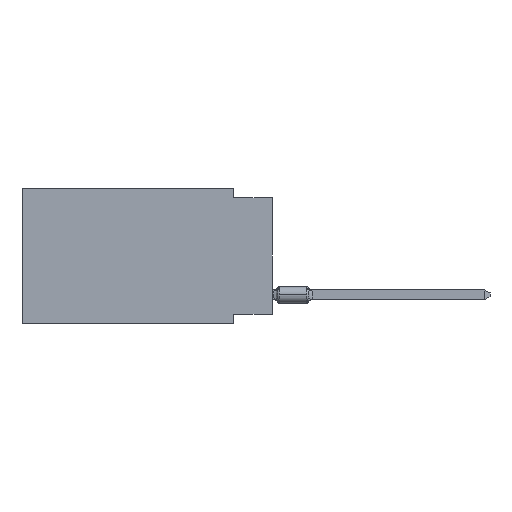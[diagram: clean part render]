
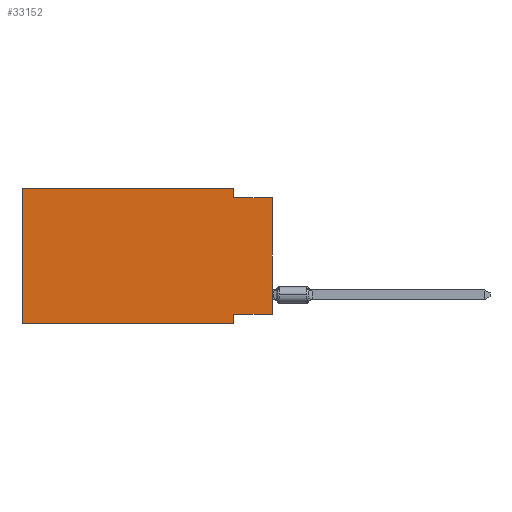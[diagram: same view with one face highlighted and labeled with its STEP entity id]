
A CAD part, left-side view. The second image highlights one B-rep face of the part: STEP entity #33152.
In plain terms, the highlighted planar face has unit normal (-1, 0, 0).
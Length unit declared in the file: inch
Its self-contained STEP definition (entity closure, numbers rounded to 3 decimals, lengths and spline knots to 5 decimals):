
#201 = VERTEX_POINT ( 'NONE', #7685 ) ;
#712 = DIRECTION ( 'NONE',  ( 0., 0., -1. ) ) ;
#1995 = EDGE_CURVE ( 'NONE', #35652, #3189, #28997, .T. ) ;
#3189 = VERTEX_POINT ( 'NONE', #18031 ) ;
#3598 = FACE_OUTER_BOUND ( 'NONE', #28103, .T. ) ;
#4036 = DIRECTION ( 'NONE',  ( 0., 0., 1. ) ) ;
#6477 = EDGE_CURVE ( 'NONE', #38400, #25236, #16079, .T. ) ;
#6953 = DIRECTION ( 'NONE',  ( 0., 0., -1. ) ) ;
#7001 = CARTESIAN_POINT ( 'NONE',  ( 0., 0.1, -0.35 ) ) ;
#7685 = CARTESIAN_POINT ( 'NONE',  ( 0., 0., -0.025 ) ) ;
#8090 = LINE ( 'NONE', #29422, #22528 ) ;
#8241 = VECTOR ( 'NONE', #712, 39.37008 ) ;
#9896 = PLANE ( 'NONE',  #38594 ) ;
#12372 = CARTESIAN_POINT ( 'NONE',  ( 0., 0.1, -0.025 ) ) ;
#12717 = DIRECTION ( 'NONE',  ( 0., -1., 0. ) ) ;
#12988 = CARTESIAN_POINT ( 'NONE',  ( 0., 0.645, 0. ) ) ;
#15323 = EDGE_CURVE ( 'NONE', #38400, #37860, #37499, .T. ) ;
#15600 = ORIENTED_EDGE ( 'NONE', *, *, #6477, .T. ) ;
#15700 = EDGE_CURVE ( 'NONE', #3189, #25236, #27212, .T. ) ;
#16079 = LINE ( 'NONE', #29769, #20965 ) ;
#16549 = ORIENTED_EDGE ( 'NONE', *, *, #17083, .F. ) ;
#17083 = EDGE_CURVE ( 'NONE', #25740, #201, #8090, .T. ) ;
#18031 = CARTESIAN_POINT ( 'NONE',  ( 0., 0.1, -0.325 ) ) ;
#18383 = VECTOR ( 'NONE', #39969, 39.37008 ) ;
#18603 = CARTESIAN_POINT ( 'NONE',  ( 0., 0.1, 0. ) ) ;
#18643 = DIRECTION ( 'NONE',  ( 0., -1., 0. ) ) ;
#19701 = EDGE_CURVE ( 'NONE', #35652, #201, #42892, .T. ) ;
#20965 = VECTOR ( 'NONE', #12717, 39.37008 ) ;
#22006 = EDGE_CURVE ( 'NONE', #24143, #25740, #39508, .T. ) ;
#22528 = VECTOR ( 'NONE', #18643, 39.37008 ) ;
#22615 = LINE ( 'NONE', #12988, #33573 ) ;
#24143 = VERTEX_POINT ( 'NONE', #18603 ) ;
#24515 = CARTESIAN_POINT ( 'NONE',  ( 0., 0.645, -0.35 ) ) ;
#25206 = CARTESIAN_POINT ( 'NONE',  ( 0., 0.1, -0.35 ) ) ;
#25236 = VERTEX_POINT ( 'NONE', #25206 ) ;
#25554 = DIRECTION ( 'NONE',  ( 0., 0., -1. ) ) ;
#25740 = VERTEX_POINT ( 'NONE', #12372 ) ;
#26337 = VECTOR ( 'NONE', #25554, 39.37008 ) ;
#26665 = DIRECTION ( 'NONE',  ( 0., -1., 0. ) ) ;
#27212 = LINE ( 'NONE', #7001, #8241 ) ;
#28103 = EDGE_LOOP ( 'NONE', ( #37641, #16549, #42723, #44230, #43222, #15600, #42569, #43515 ) ) ;
#28997 = LINE ( 'NONE', #36186, #42682 ) ;
#29422 = CARTESIAN_POINT ( 'NONE',  ( 0., 0., -0.025 ) ) ;
#29769 = CARTESIAN_POINT ( 'NONE',  ( 0., 0.645, -0.35 ) ) ;
#32301 = CARTESIAN_POINT ( 'NONE',  ( 0., 0.645, 0. ) ) ;
#33152 = ADVANCED_FACE ( 'NONE', ( #3598 ), #9896, .F. ) ;
#33392 = VECTOR ( 'NONE', #4036, 39.37008 ) ;
#33573 = VECTOR ( 'NONE', #26665, 39.37008 ) ;
#33597 = EDGE_CURVE ( 'NONE', #37860, #24143, #22615, .T. ) ;
#34589 = CARTESIAN_POINT ( 'NONE',  ( 0., 0.645, 0. ) ) ;
#35225 = CARTESIAN_POINT ( 'NONE',  ( 0., 0.645, 0. ) ) ;
#35652 = VERTEX_POINT ( 'NONE', #42721 ) ;
#36186 = CARTESIAN_POINT ( 'NONE',  ( 0., 0., -0.325 ) ) ;
#36370 = CARTESIAN_POINT ( 'NONE',  ( 0., 0., 0. ) ) ;
#37499 = LINE ( 'NONE', #35225, #33392 ) ;
#37641 = ORIENTED_EDGE ( 'NONE', *, *, #19701, .T. ) ;
#37726 = DIRECTION ( 'NONE',  ( 1., 0., 0. ) ) ;
#37860 = VERTEX_POINT ( 'NONE', #32301 ) ;
#38400 = VERTEX_POINT ( 'NONE', #24515 ) ;
#38594 = AXIS2_PLACEMENT_3D ( 'NONE', #34589, #37726, #6953 ) ;
#38844 = CARTESIAN_POINT ( 'NONE',  ( 0., 0.1, 0. ) ) ;
#39508 = LINE ( 'NONE', #38844, #26337 ) ;
#39969 = DIRECTION ( 'NONE',  ( 0., 0., 1. ) ) ;
#42569 = ORIENTED_EDGE ( 'NONE', *, *, #15700, .F. ) ;
#42682 = VECTOR ( 'NONE', #42700, 39.37008 ) ;
#42700 = DIRECTION ( 'NONE',  ( 0., 1., 0. ) ) ;
#42721 = CARTESIAN_POINT ( 'NONE',  ( 0., 0., -0.325 ) ) ;
#42723 = ORIENTED_EDGE ( 'NONE', *, *, #22006, .F. ) ;
#42892 = LINE ( 'NONE', #36370, #18383 ) ;
#43222 = ORIENTED_EDGE ( 'NONE', *, *, #15323, .F. ) ;
#43515 = ORIENTED_EDGE ( 'NONE', *, *, #1995, .F. ) ;
#44230 = ORIENTED_EDGE ( 'NONE', *, *, #33597, .F. ) ;
